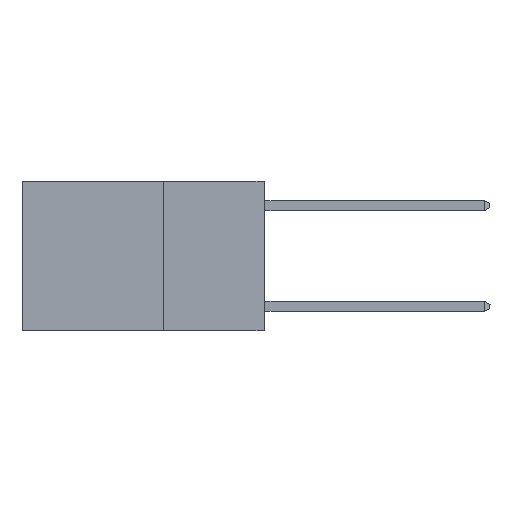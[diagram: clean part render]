
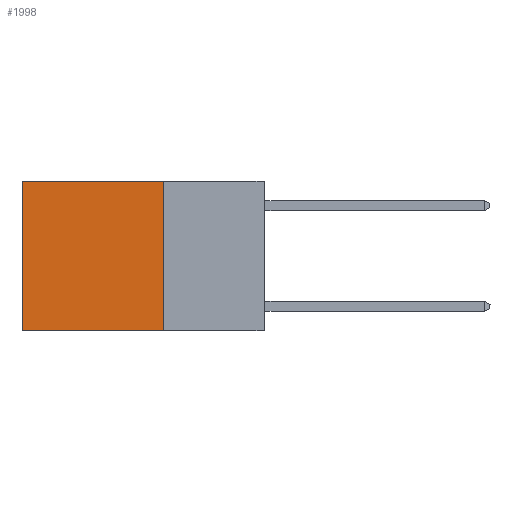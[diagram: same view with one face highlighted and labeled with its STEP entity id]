
A CAD part, left-side view. The second image highlights one B-rep face of the part: STEP entity #1998.
In plain terms, the highlighted planar face has unit normal (-1, 0, 0).
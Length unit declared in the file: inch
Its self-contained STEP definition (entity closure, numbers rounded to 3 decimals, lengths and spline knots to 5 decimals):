
#57 = EDGE_CURVE ( 'NONE', #7215, #6332, #3876, .T. ) ;
#1549 = CARTESIAN_POINT ( 'NONE',  ( 0.2625, 0.6, 0. ) ) ;
#1587 = EDGE_CURVE ( 'NONE', #7215, #8537, #2936, .T. ) ;
#1998 = ADVANCED_FACE ( 'NONE', ( #6320 ), #8605, .F. ) ;
#2222 = ORIENTED_EDGE ( 'NONE', *, *, #5769, .T. ) ;
#2447 = ORIENTED_EDGE ( 'NONE', *, *, #4692, .F. ) ;
#2463 = ORIENTED_EDGE ( 'NONE', *, *, #1587, .F. ) ;
#2584 = ORIENTED_EDGE ( 'NONE', *, *, #57, .T. ) ;
#2936 = LINE ( 'NONE', #8625, #8920 ) ;
#3129 = VERTEX_POINT ( 'NONE', #3687 ) ;
#3437 = DIRECTION ( 'NONE',  ( 0., 1., 0. ) ) ;
#3687 = CARTESIAN_POINT ( 'NONE',  ( 0.2625, 0.6, -0.37 ) ) ;
#3764 = CARTESIAN_POINT ( 'NONE',  ( 0.2625, 0.25, 0. ) ) ;
#3876 = LINE ( 'NONE', #3764, #7788 ) ;
#4636 = CARTESIAN_POINT ( 'NONE',  ( 0.2625, 0.25, 0. ) ) ;
#4692 = EDGE_CURVE ( 'NONE', #8537, #3129, #6136, .T. ) ;
#4846 = CARTESIAN_POINT ( 'NONE',  ( 0.2625, 0.25, 0. ) ) ;
#5716 = DIRECTION ( 'NONE',  ( 0., 0., -1. ) ) ;
#5732 = LINE ( 'NONE', #8325, #9336 ) ;
#5769 = EDGE_CURVE ( 'NONE', #6332, #3129, #5732, .T. ) ;
#5953 = CARTESIAN_POINT ( 'NONE',  ( 0.2625, 0.25, -0.37 ) ) ;
#6136 = LINE ( 'NONE', #5953, #6369 ) ;
#6320 = FACE_OUTER_BOUND ( 'NONE', #8546, .T. ) ;
#6332 = VERTEX_POINT ( 'NONE', #1549 ) ;
#6369 = VECTOR ( 'NONE', #3437, 39.37008 ) ;
#7183 = DIRECTION ( 'NONE',  ( 0., 1., 0. ) ) ;
#7215 = VERTEX_POINT ( 'NONE', #4636 ) ;
#7242 = AXIS2_PLACEMENT_3D ( 'NONE', #4846, #10000, #5716 ) ;
#7750 = CARTESIAN_POINT ( 'NONE',  ( 0.2625, 0.25, -0.37 ) ) ;
#7788 = VECTOR ( 'NONE', #7183, 39.37008 ) ;
#8258 = DIRECTION ( 'NONE',  ( 0., 0., -1. ) ) ;
#8325 = CARTESIAN_POINT ( 'NONE',  ( 0.2625, 0.6, 0. ) ) ;
#8537 = VERTEX_POINT ( 'NONE', #7750 ) ;
#8546 = EDGE_LOOP ( 'NONE', ( #2222, #2447, #2463, #2584 ) ) ;
#8605 = PLANE ( 'NONE',  #7242 ) ;
#8625 = CARTESIAN_POINT ( 'NONE',  ( 0.2625, 0.25, 0. ) ) ;
#8920 = VECTOR ( 'NONE', #8258, 39.37008 ) ;
#9051 = DIRECTION ( 'NONE',  ( 0., 0., -1. ) ) ;
#9336 = VECTOR ( 'NONE', #9051, 39.37008 ) ;
#10000 = DIRECTION ( 'NONE',  ( 1., 0., 0. ) ) ;
